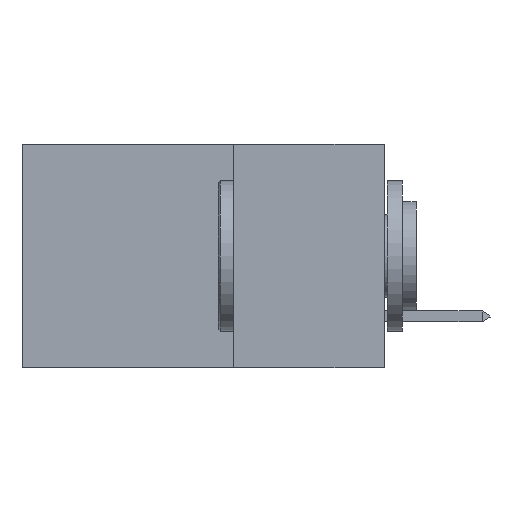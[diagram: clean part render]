
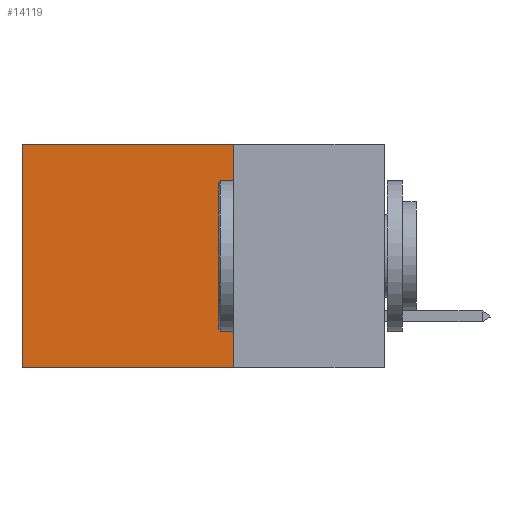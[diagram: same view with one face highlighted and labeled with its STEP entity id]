
A CAD part, left-side view. The second image highlights one B-rep face of the part: STEP entity #14119.
In plain terms, the highlighted planar face has unit normal (-1, 0, 0).
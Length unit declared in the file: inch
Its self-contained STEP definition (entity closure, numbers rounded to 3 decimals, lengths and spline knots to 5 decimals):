
#138 = LINE ( 'NONE', #6356, #38423 ) ;
#2194 = FACE_OUTER_BOUND ( 'NONE', #7640, .T. ) ;
#3475 = DIRECTION ( 'NONE',  ( 0., 1., 0. ) ) ;
#4093 = CARTESIAN_POINT ( 'NONE',  ( 0.2875, 0.25, 0. ) ) ;
#5002 = CARTESIAN_POINT ( 'NONE',  ( 0.2875, 0.6, -0.37 ) ) ;
#5023 = VECTOR ( 'NONE', #3475, 39.37008 ) ;
#5579 = VECTOR ( 'NONE', #7038, 39.37008 ) ;
#5619 = PLANE ( 'NONE',  #7988 ) ;
#6356 = CARTESIAN_POINT ( 'NONE',  ( 0.2875, 0.25, -0.37 ) ) ;
#7038 = DIRECTION ( 'NONE',  ( 0., 0., -1. ) ) ;
#7499 = LINE ( 'NONE', #18942, #5023 ) ;
#7640 = EDGE_LOOP ( 'NONE', ( #35843, #26055, #29047, #12402 ) ) ;
#7955 = VERTEX_POINT ( 'NONE', #23302 ) ;
#7988 = AXIS2_PLACEMENT_3D ( 'NONE', #44911, #9709, #21676 ) ;
#9709 = DIRECTION ( 'NONE',  ( 1., 0., 0. ) ) ;
#12402 = ORIENTED_EDGE ( 'NONE', *, *, #26392, .T. ) ;
#13594 = VERTEX_POINT ( 'NONE', #40744 ) ;
#14119 = ADVANCED_FACE ( 'NONE', ( #2194 ), #5619, .F. ) ;
#14336 = CARTESIAN_POINT ( 'NONE',  ( 0.2875, 0.6, 0. ) ) ;
#16794 = EDGE_CURVE ( 'NONE', #27355, #42215, #40163, .T. ) ;
#17098 = VECTOR ( 'NONE', #43252, 39.37008 ) ;
#18942 = CARTESIAN_POINT ( 'NONE',  ( 0.2875, 0.25, 0. ) ) ;
#21644 = CARTESIAN_POINT ( 'NONE',  ( 0.2875, 0.6, 0. ) ) ;
#21676 = DIRECTION ( 'NONE',  ( 0., 0., -1. ) ) ;
#23302 = CARTESIAN_POINT ( 'NONE',  ( 0.2875, 0.25, -0.37 ) ) ;
#23857 = EDGE_CURVE ( 'NONE', #7955, #42215, #138, .T. ) ;
#26055 = ORIENTED_EDGE ( 'NONE', *, *, #23857, .F. ) ;
#26392 = EDGE_CURVE ( 'NONE', #13594, #27355, #7499, .T. ) ;
#27355 = VERTEX_POINT ( 'NONE', #21644 ) ;
#29047 = ORIENTED_EDGE ( 'NONE', *, *, #40856, .F. ) ;
#33441 = DIRECTION ( 'NONE',  ( 0., 1., 0. ) ) ;
#35254 = LINE ( 'NONE', #4093, #17098 ) ;
#35843 = ORIENTED_EDGE ( 'NONE', *, *, #16794, .T. ) ;
#38423 = VECTOR ( 'NONE', #33441, 39.37008 ) ;
#40163 = LINE ( 'NONE', #14336, #5579 ) ;
#40744 = CARTESIAN_POINT ( 'NONE',  ( 0.2875, 0.25, 0. ) ) ;
#40856 = EDGE_CURVE ( 'NONE', #13594, #7955, #35254, .T. ) ;
#42215 = VERTEX_POINT ( 'NONE', #5002 ) ;
#43252 = DIRECTION ( 'NONE',  ( 0., 0., -1. ) ) ;
#44911 = CARTESIAN_POINT ( 'NONE',  ( 0.2875, 0.25, 0. ) ) ;
